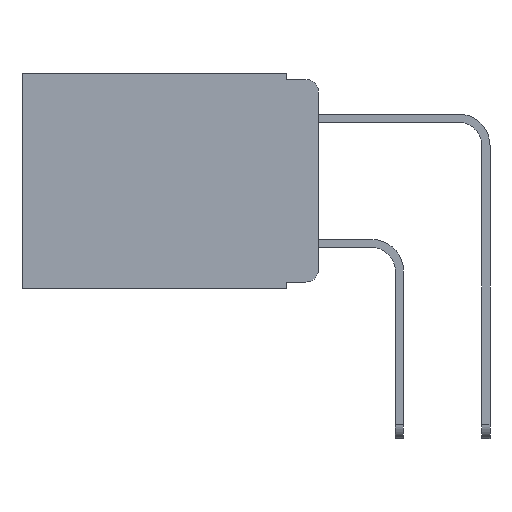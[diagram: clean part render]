
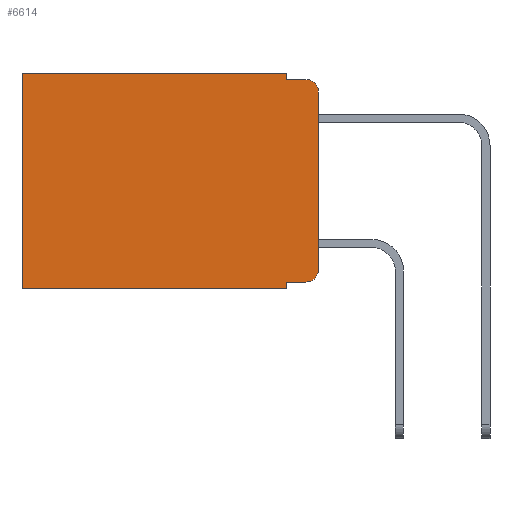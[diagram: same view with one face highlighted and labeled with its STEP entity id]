
A CAD part, left-side view. The second image highlights one B-rep face of the part: STEP entity #6614.
In plain terms, the highlighted planar face has unit normal (-1, 0, 0).
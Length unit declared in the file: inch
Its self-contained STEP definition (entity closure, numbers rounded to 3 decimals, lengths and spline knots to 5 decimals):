
#103 = EDGE_CURVE ( 'NONE', #4167, #11408, #11683, .T. ) ;
#153 = VERTEX_POINT ( 'NONE', #2837 ) ;
#243 = VERTEX_POINT ( 'NONE', #10668 ) ;
#344 = CARTESIAN_POINT ( 'NONE',  ( 0.298, 0.051, -0.01 ) ) ;
#531 = LINE ( 'NONE', #8729, #2880 ) ;
#603 = VECTOR ( 'NONE', #7678, 39.37008 ) ;
#705 = CARTESIAN_POINT ( 'NONE',  ( 0.298, 0., -0.313 ) ) ;
#906 = VECTOR ( 'NONE', #11946, 39.37008 ) ;
#1047 = EDGE_CURVE ( 'NONE', #153, #243, #9903, .T. ) ;
#1240 = VERTEX_POINT ( 'NONE', #5593 ) ;
#1695 = VERTEX_POINT ( 'NONE', #705 ) ;
#1919 = VERTEX_POINT ( 'NONE', #10404 ) ;
#2145 = LINE ( 'NONE', #8769, #2458 ) ;
#2292 = CARTESIAN_POINT ( 'NONE',  ( 0.298, 0.051, 0. ) ) ;
#2309 = CARTESIAN_POINT ( 'NONE',  ( 0.298, 0.473, 0. ) ) ;
#2458 = VECTOR ( 'NONE', #3885, 39.37008 ) ;
#2568 = EDGE_CURVE ( 'NONE', #10754, #7131, #2145, .T. ) ;
#2837 = CARTESIAN_POINT ( 'NONE',  ( 0.298, 0., -0.03 ) ) ;
#2880 = VECTOR ( 'NONE', #3883, 39.37008 ) ;
#2938 = DIRECTION ( 'NONE',  ( -1., 0., 0. ) ) ;
#3031 = CARTESIAN_POINT ( 'NONE',  ( 0.298, 0., 0. ) ) ;
#3123 = VECTOR ( 'NONE', #8866, 39.37008 ) ;
#3135 = ORIENTED_EDGE ( 'NONE', *, *, #2568, .T. ) ;
#3734 = EDGE_LOOP ( 'NONE', ( #4372, #10969, #9614, #6146, #6170, #6544, #4908, #6542, #3135, #9628 ) ) ;
#3883 = DIRECTION ( 'NONE',  ( 0., 0., -1. ) ) ;
#3885 = DIRECTION ( 'NONE',  ( 0., -1., 0. ) ) ;
#3966 = AXIS2_PLACEMENT_3D ( 'NONE', #8518, #2938, #9422 ) ;
#4167 = VERTEX_POINT ( 'NONE', #8650 ) ;
#4260 = AXIS2_PLACEMENT_3D ( 'NONE', #10024, #8539, #11849 ) ;
#4372 = ORIENTED_EDGE ( 'NONE', *, *, #6464, .F. ) ;
#4818 = VECTOR ( 'NONE', #8763, 39.37008 ) ;
#4906 = CARTESIAN_POINT ( 'NONE',  ( 0.298, 0.02, -0.333 ) ) ;
#4908 = ORIENTED_EDGE ( 'NONE', *, *, #12039, .F. ) ;
#4986 = EDGE_CURVE ( 'NONE', #11408, #243, #7268, .T. ) ;
#5055 = DIRECTION ( 'NONE',  ( 0., 1., 0. ) ) ;
#5329 = VECTOR ( 'NONE', #5055, 39.37008 ) ;
#5593 = CARTESIAN_POINT ( 'NONE',  ( 0.298, 0.051, -0.343 ) ) ;
#5668 = LINE ( 'NONE', #2309, #3123 ) ;
#5803 = LINE ( 'NONE', #3031, #603 ) ;
#5936 = VERTEX_POINT ( 'NONE', #8195 ) ;
#6076 = LINE ( 'NONE', #11094, #906 ) ;
#6146 = ORIENTED_EDGE ( 'NONE', *, *, #103, .F. ) ;
#6170 = ORIENTED_EDGE ( 'NONE', *, *, #10269, .T. ) ;
#6202 = CARTESIAN_POINT ( 'NONE',  ( 0.298, 0.02, -0.03 ) ) ;
#6445 = FACE_OUTER_BOUND ( 'NONE', #3734, .T. ) ;
#6464 = EDGE_CURVE ( 'NONE', #153, #1695, #531, .T. ) ;
#6542 = ORIENTED_EDGE ( 'NONE', *, *, #11395, .F. ) ;
#6544 = ORIENTED_EDGE ( 'NONE', *, *, #9057, .T. ) ;
#6614 = ADVANCED_FACE ( 'NONE', ( #6445 ), #8627, .F. ) ;
#6826 = AXIS2_PLACEMENT_3D ( 'NONE', #6202, #8263, #11309 ) ;
#7131 = VERTEX_POINT ( 'NONE', #4906 ) ;
#7268 = LINE ( 'NONE', #344, #4818 ) ;
#7528 = CARTESIAN_POINT ( 'NONE',  ( 0.298, 0.051, -0.01 ) ) ;
#7678 = DIRECTION ( 'NONE',  ( 0., 1., 0. ) ) ;
#7919 = DIRECTION ( 'NONE',  ( 0., 0., -1. ) ) ;
#8034 = LINE ( 'NONE', #8697, #5329 ) ;
#8195 = CARTESIAN_POINT ( 'NONE',  ( 0.298, 0.473, -0.343 ) ) ;
#8209 = EDGE_CURVE ( 'NONE', #7131, #1695, #10201, .T. ) ;
#8263 = DIRECTION ( 'NONE',  ( -1., 0., 0. ) ) ;
#8365 = CARTESIAN_POINT ( 'NONE',  ( 0.298, 0.051, -0.333 ) ) ;
#8518 = CARTESIAN_POINT ( 'NONE',  ( 0.298, 0.02, -0.313 ) ) ;
#8539 = DIRECTION ( 'NONE',  ( 1., 0., 0. ) ) ;
#8627 = PLANE ( 'NONE',  #4260 ) ;
#8650 = CARTESIAN_POINT ( 'NONE',  ( 0.298, 0.051, 0. ) ) ;
#8697 = CARTESIAN_POINT ( 'NONE',  ( 0.298, 0., -0.343 ) ) ;
#8729 = CARTESIAN_POINT ( 'NONE',  ( 0.298, 0., 0. ) ) ;
#8763 = DIRECTION ( 'NONE',  ( 0., -1., 0. ) ) ;
#8769 = CARTESIAN_POINT ( 'NONE',  ( 0.298, 0.051, -0.333 ) ) ;
#8866 = DIRECTION ( 'NONE',  ( 0., 0., -1. ) ) ;
#9057 = EDGE_CURVE ( 'NONE', #1919, #5936, #5668, .T. ) ;
#9369 = VECTOR ( 'NONE', #7919, 39.37008 ) ;
#9422 = DIRECTION ( 'NONE',  ( 0., 0., -1. ) ) ;
#9614 = ORIENTED_EDGE ( 'NONE', *, *, #4986, .F. ) ;
#9628 = ORIENTED_EDGE ( 'NONE', *, *, #8209, .T. ) ;
#9903 = CIRCLE ( 'NONE', #6826, 0.02 ) ;
#10024 = CARTESIAN_POINT ( 'NONE',  ( 0.298, 0., 0. ) ) ;
#10201 = CIRCLE ( 'NONE', #3966, 0.02 ) ;
#10269 = EDGE_CURVE ( 'NONE', #4167, #1919, #5803, .T. ) ;
#10404 = CARTESIAN_POINT ( 'NONE',  ( 0.298, 0.473, 0. ) ) ;
#10668 = CARTESIAN_POINT ( 'NONE',  ( 0.298, 0.02, -0.01 ) ) ;
#10754 = VERTEX_POINT ( 'NONE', #8365 ) ;
#10969 = ORIENTED_EDGE ( 'NONE', *, *, #1047, .T. ) ;
#11094 = CARTESIAN_POINT ( 'NONE',  ( 0.298, 0.051, 0. ) ) ;
#11309 = DIRECTION ( 'NONE',  ( 0., 0., -1. ) ) ;
#11395 = EDGE_CURVE ( 'NONE', #10754, #1240, #6076, .T. ) ;
#11408 = VERTEX_POINT ( 'NONE', #7528 ) ;
#11683 = LINE ( 'NONE', #2292, #9369 ) ;
#11849 = DIRECTION ( 'NONE',  ( 0., 0., -1. ) ) ;
#11946 = DIRECTION ( 'NONE',  ( 0., 0., -1. ) ) ;
#12039 = EDGE_CURVE ( 'NONE', #1240, #5936, #8034, .T. ) ;
